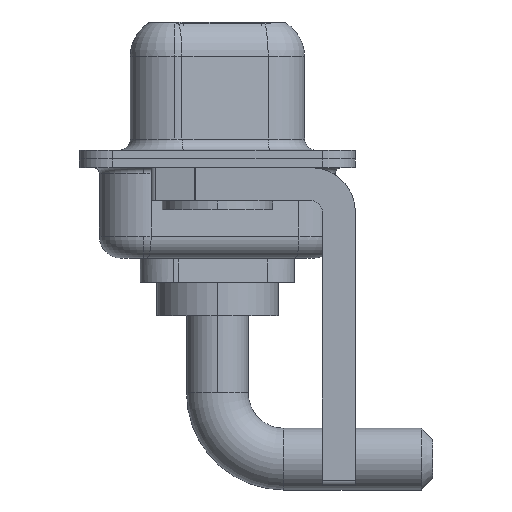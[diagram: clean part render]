
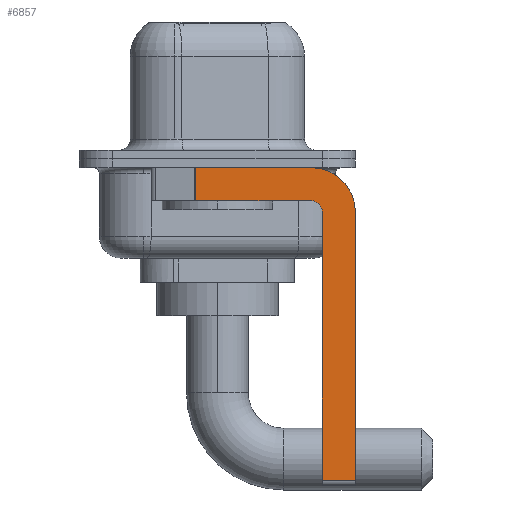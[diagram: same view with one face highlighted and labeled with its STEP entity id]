
A CAD part, left-side view. The second image highlights one B-rep face of the part: STEP entity #6857.
In plain terms, the highlighted planar face has unit normal (-1, 0, 0).
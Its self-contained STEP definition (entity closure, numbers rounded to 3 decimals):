
#319 = EDGE_LOOP ( 'NONE', ( #4180, #7471, #4964, #8822, #6711, #5190, #7757, #637 ) ) ;
#637 = ORIENTED_EDGE ( 'NONE', *, *, #5443, .F. ) ;
#686 = EDGE_CURVE ( 'NONE', #12407, #7497, #2146, .T. ) ;
#708 = VERTEX_POINT ( 'NONE', #12262 ) ;
#1288 = DIRECTION ( 'NONE',  ( 0., 1., 0. ) ) ;
#1350 = AXIS2_PLACEMENT_3D ( 'NONE', #2454, #6462, #10429 ) ;
#1356 = EDGE_CURVE ( 'NONE', #7430, #708, #7610, .T. ) ;
#1357 = VECTOR ( 'NONE', #4488, 1000. ) ;
#1480 = EDGE_CURVE ( 'NONE', #8566, #708, #4924, .T. ) ;
#1608 = LINE ( 'NONE', #6459, #1357 ) ;
#1626 = EDGE_CURVE ( 'NONE', #3180, #7497, #4194, .T. ) ;
#1777 = CIRCLE ( 'NONE', #11361, 2. ) ;
#1919 = CARTESIAN_POINT ( 'NONE',  ( -2.9, -4.25, -2.4 ) ) ;
#2043 = DIRECTION ( 'NONE',  ( 0., 0., -1. ) ) ;
#2146 = LINE ( 'NONE', #12067, #8997 ) ;
#2454 = CARTESIAN_POINT ( 'NONE',  ( -2.9, -4.25, -2.4 ) ) ;
#3180 = VERTEX_POINT ( 'NONE', #9645 ) ;
#3436 = FACE_OUTER_BOUND ( 'NONE', #319, .T. ) ;
#3463 = DIRECTION ( 'NONE',  ( 0., 0., 1. ) ) ;
#3684 = CARTESIAN_POINT ( 'NONE',  ( -2.9, 0.978, -1.9 ) ) ;
#3769 = CARTESIAN_POINT ( 'NONE',  ( -2.9, -4.75, -14.55 ) ) ;
#3799 = CARTESIAN_POINT ( 'NONE',  ( -2.9, -4.75, -14.8 ) ) ;
#3913 = EDGE_CURVE ( 'NONE', #11787, #12407, #4883, .T. ) ;
#4180 = ORIENTED_EDGE ( 'NONE', *, *, #11488, .F. ) ;
#4194 = LINE ( 'NONE', #4328, #9424 ) ;
#4205 = CARTESIAN_POINT ( 'NONE',  ( -2.9, -6.25, -2.4 ) ) ;
#4328 = CARTESIAN_POINT ( 'NONE',  ( -2.9, 0.978, -1.9 ) ) ;
#4488 = DIRECTION ( 'NONE',  ( 0., -1., 0. ) ) ;
#4883 = CIRCLE ( 'NONE', #7601, 0.5 ) ;
#4924 = LINE ( 'NONE', #12081, #6942 ) ;
#4964 = ORIENTED_EDGE ( 'NONE', *, *, #686, .F. ) ;
#4984 = DIRECTION ( 'NONE',  ( 1., 0., 0. ) ) ;
#5178 = DIRECTION ( 'NONE',  ( 0., 0., -1. ) ) ;
#5190 = ORIENTED_EDGE ( 'NONE', *, *, #1356, .T. ) ;
#5443 = EDGE_CURVE ( 'NONE', #10084, #8566, #1777, .T. ) ;
#5610 = VECTOR ( 'NONE', #11760, 1000. ) ;
#5712 = CARTESIAN_POINT ( 'NONE',  ( -2.9, -4.25, -14.55 ) ) ;
#6459 = CARTESIAN_POINT ( 'NONE',  ( -2.9, 3., -0.4 ) ) ;
#6462 = DIRECTION ( 'NONE',  ( 1., 0., 0. ) ) ;
#6711 = ORIENTED_EDGE ( 'NONE', *, *, #8920, .F. ) ;
#6857 = ADVANCED_FACE ( 'NONE', ( #3436 ), #11409, .F. ) ;
#6942 = VECTOR ( 'NONE', #2043, 1000. ) ;
#7430 = VERTEX_POINT ( 'NONE', #3769 ) ;
#7471 = ORIENTED_EDGE ( 'NONE', *, *, #1626, .T. ) ;
#7497 = VERTEX_POINT ( 'NONE', #3684 ) ;
#7601 = AXIS2_PLACEMENT_3D ( 'NONE', #1919, #9688, #3463 ) ;
#7610 = LINE ( 'NONE', #5712, #7759 ) ;
#7757 = ORIENTED_EDGE ( 'NONE', *, *, #1480, .F. ) ;
#7759 = VECTOR ( 'NONE', #11582, 1000. ) ;
#7932 = LINE ( 'NONE', #3799, #5610 ) ;
#8566 = VERTEX_POINT ( 'NONE', #4205 ) ;
#8619 = CARTESIAN_POINT ( 'NONE',  ( -2.9, -4.25, -2.4 ) ) ;
#8822 = ORIENTED_EDGE ( 'NONE', *, *, #3913, .F. ) ;
#8920 = EDGE_CURVE ( 'NONE', #7430, #11787, #7932, .T. ) ;
#8997 = VECTOR ( 'NONE', #1288, 1000. ) ;
#9424 = VECTOR ( 'NONE', #5178, 1000. ) ;
#9585 = DIRECTION ( 'NONE',  ( 0., 0., -1. ) ) ;
#9645 = CARTESIAN_POINT ( 'NONE',  ( -2.9, 0.978, -0.4 ) ) ;
#9688 = DIRECTION ( 'NONE',  ( -1., 0., 0. ) ) ;
#10042 = CARTESIAN_POINT ( 'NONE',  ( -2.9, -4.75, -2.4 ) ) ;
#10084 = VERTEX_POINT ( 'NONE', #12191 ) ;
#10429 = DIRECTION ( 'NONE',  ( 0., 0., -1. ) ) ;
#10663 = CARTESIAN_POINT ( 'NONE',  ( -2.9, -4.25, -1.9 ) ) ;
#11361 = AXIS2_PLACEMENT_3D ( 'NONE', #8619, #4984, #9585 ) ;
#11409 = PLANE ( 'NONE',  #1350 ) ;
#11488 = EDGE_CURVE ( 'NONE', #3180, #10084, #1608, .T. ) ;
#11582 = DIRECTION ( 'NONE',  ( 0., -1., 0. ) ) ;
#11760 = DIRECTION ( 'NONE',  ( 0., 0., 1. ) ) ;
#11787 = VERTEX_POINT ( 'NONE', #10042 ) ;
#12067 = CARTESIAN_POINT ( 'NONE',  ( -2.9, -4.25, -1.9 ) ) ;
#12081 = CARTESIAN_POINT ( 'NONE',  ( -2.9, -6.25, -2.4 ) ) ;
#12191 = CARTESIAN_POINT ( 'NONE',  ( -2.9, -4.25, -0.4 ) ) ;
#12262 = CARTESIAN_POINT ( 'NONE',  ( -2.9, -6.25, -14.55 ) ) ;
#12407 = VERTEX_POINT ( 'NONE', #10663 ) ;
